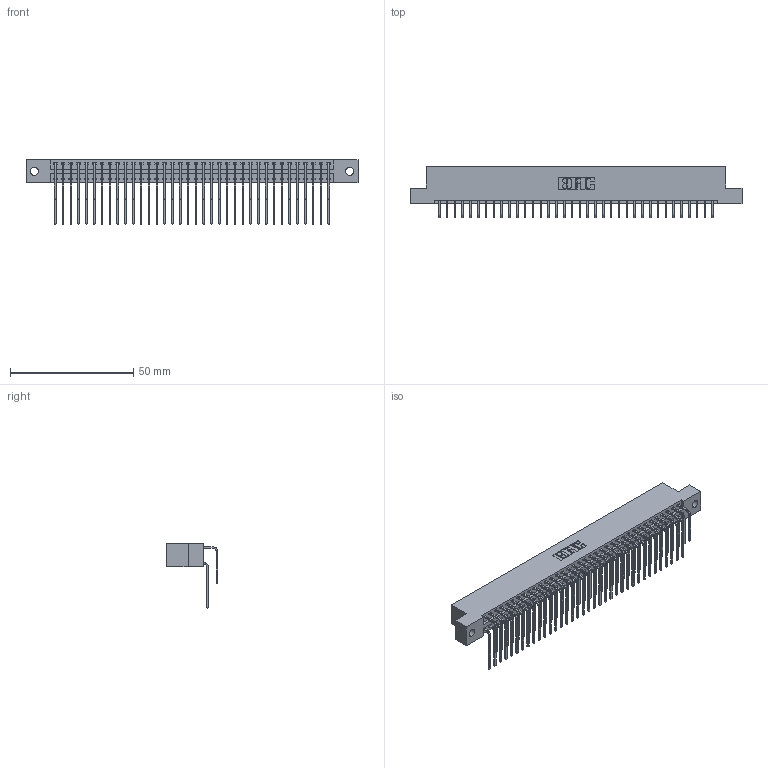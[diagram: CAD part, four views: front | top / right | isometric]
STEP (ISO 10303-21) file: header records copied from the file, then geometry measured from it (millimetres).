
FILE_DESCRIPTION (( 'STEP AP203' ), '1' );
FILE_NAME ('346-072-559-202.STEP', '2022-05-25T00:57:11', ( '' ), ( '' ), 'SwSTEP 2.0', 'SolidWorks 2020', '' );
FILE_SCHEMA (( 'CONFIG_CONTROL_DESIGN' ));
Length unit declared in the file: inch
Products named in the file (4): 345-292-001_559 Tail - 2; 345-292-001_558 559 Tail - 1; 346 Part_Flush Mounting Lugs - 0.128 Dia; 346-072-559-202
Assembly tree (73 placements, depth 2):
  346-072-559-202
    346 Part_Flush Mounting Lugs - 0.128 Dia
    345-292-001_558 559 Tail - 1  x36
    345-292-001_559 Tail - 2  x36
Bounding box: 134.87 x 20.89 x 26.16 mm (x, y, z)
Volume: 13484 mm3; surface area: 20163.6 mm2
Topology: 73 solids, 73 shells, 4010 faces, 11921 edges, 7850 vertices
Faces by surface type: plane 2740, cylinder 1270
Entity records: 26089 total; most frequent: CARTESIAN_POINT 4359, ORIENTED_EDGE 4242, DIRECTION 3865, EDGE_CURVE 2121, LINE 1805, VECTOR 1805, VERTEX_POINT 1410, AXIS2_PLACEMENT_3D 1030
